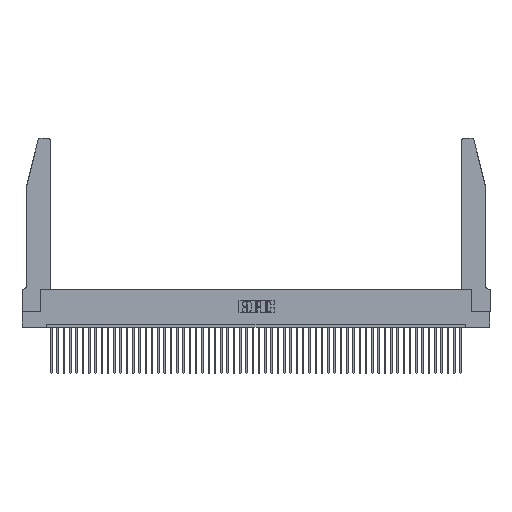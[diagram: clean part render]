
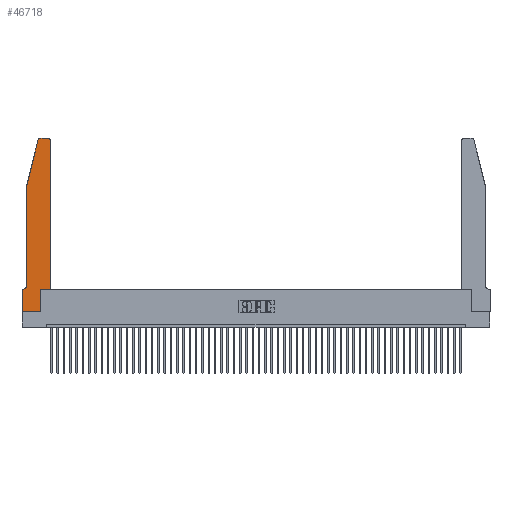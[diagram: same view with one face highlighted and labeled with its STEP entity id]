
A CAD part, top view. The second image highlights one B-rep face of the part: STEP entity #46718.
In plain terms, the highlighted planar face has unit normal (0, 0, 1).
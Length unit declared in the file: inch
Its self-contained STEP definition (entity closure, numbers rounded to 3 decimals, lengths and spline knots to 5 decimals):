
#19 = DIRECTION ( 'NONE',  ( 0., 0., 1. ) ) ;
#171 = EDGE_CURVE ( 'NONE', #25210, #6181, #39490, .T. ) ;
#871 = CARTESIAN_POINT ( 'NONE',  ( 0.2865, 0.35, 0.37 ) ) ;
#1043 = DIRECTION ( 'NONE',  ( 0., 1., 0. ) ) ;
#1110 = VERTEX_POINT ( 'NONE', #12302 ) ;
#1842 = ORIENTED_EDGE ( 'NONE', *, *, #15067, .T. ) ;
#2196 = CARTESIAN_POINT ( 'NONE',  ( 0., 0.35, 0.37 ) ) ;
#2297 = VECTOR ( 'NONE', #5967, 39.37008 ) ;
#3473 = LINE ( 'NONE', #14697, #22764 ) ;
#3910 = DIRECTION ( 'NONE',  ( 0., -1., 0. ) ) ;
#4078 = ORIENTED_EDGE ( 'NONE', *, *, #33581, .T. ) ;
#4260 = EDGE_CURVE ( 'NONE', #44697, #17746, #29826, .T. ) ;
#4726 = CARTESIAN_POINT ( 'NONE',  ( 0., 0., 0.37 ) ) ;
#5235 = VERTEX_POINT ( 'NONE', #29947 ) ;
#5526 = DIRECTION ( 'NONE',  ( 1., 0., 0. ) ) ;
#5967 = DIRECTION ( 'NONE',  ( -1., 0., 0. ) ) ;
#6181 = VERTEX_POINT ( 'NONE', #27707 ) ;
#7035 = ORIENTED_EDGE ( 'NONE', *, *, #21405, .T. ) ;
#7250 = EDGE_CURVE ( 'NONE', #1110, #44697, #3473, .T. ) ;
#7410 = VECTOR ( 'NONE', #10769, 39.37008 ) ;
#8171 = DIRECTION ( 'NONE',  ( 1., 0., 0. ) ) ;
#8192 = CARTESIAN_POINT ( 'NONE',  ( 0.4505, 0.35, 0.37 ) ) ;
#9369 = DIRECTION ( 'NONE',  ( 0., 1., 0. ) ) ;
#9827 = VECTOR ( 'NONE', #3910, 39.37008 ) ;
#10769 = DIRECTION ( 'NONE',  ( 1., 0., 0. ) ) ;
#12302 = CARTESIAN_POINT ( 'NONE',  ( 0.0055, 0.35, 0.37 ) ) ;
#13130 = CARTESIAN_POINT ( 'NONE',  ( 0.0055, 0.42, 0.37 ) ) ;
#13409 = CARTESIAN_POINT ( 'NONE',  ( 0.0755, 2., 0.37 ) ) ;
#13596 = CARTESIAN_POINT ( 'NONE',  ( 0., 0., 0.37 ) ) ;
#13872 = ORIENTED_EDGE ( 'NONE', *, *, #24236, .T. ) ;
#14280 = CARTESIAN_POINT ( 'NONE',  ( 0.2605, 2.75, 0.37 ) ) ;
#14697 = CARTESIAN_POINT ( 'NONE',  ( 0.0755, 0.35, 0.37 ) ) ;
#15067 = EDGE_CURVE ( 'NONE', #46160, #40145, #40225, .T. ) ;
#15393 = CIRCLE ( 'NONE', #32398, 0.07 ) ;
#15553 = VERTEX_POINT ( 'NONE', #37502 ) ;
#15912 = CARTESIAN_POINT ( 'NONE',  ( 0., 0.35, 0.37 ) ) ;
#16019 = EDGE_CURVE ( 'NONE', #15553, #5235, #30978, .T. ) ;
#16510 = LINE ( 'NONE', #41468, #25239 ) ;
#16711 = VERTEX_POINT ( 'NONE', #38688 ) ;
#17746 = VERTEX_POINT ( 'NONE', #13596 ) ;
#18865 = LINE ( 'NONE', #871, #36101 ) ;
#19249 = AXIS2_PLACEMENT_3D ( 'NONE', #21527, #39036, #47330 ) ;
#19499 = CARTESIAN_POINT ( 'NONE',  ( 0.25487, 2.72718, 0.37 ) ) ;
#20459 = ORIENTED_EDGE ( 'NONE', *, *, #16019, .T. ) ;
#20524 = EDGE_LOOP ( 'NONE', ( #37346, #1842, #40385, #47467, #13872, #21397, #48503, #25365, #7035, #20459, #44644, #4078 ) ) ;
#20761 = DIRECTION ( 'NONE',  ( 0., 0., -1. ) ) ;
#20930 = DIRECTION ( 'NONE',  ( -1., 0., 0. ) ) ;
#21397 = ORIENTED_EDGE ( 'NONE', *, *, #7250, .T. ) ;
#21405 = EDGE_CURVE ( 'NONE', #16711, #15553, #18865, .T. ) ;
#21527 = CARTESIAN_POINT ( 'NONE',  ( 0.4205, 2.72, 0.37 ) ) ;
#22764 = VECTOR ( 'NONE', #42815, 39.37008 ) ;
#23210 = AXIS2_PLACEMENT_3D ( 'NONE', #28275, #47425, #8171 ) ;
#24236 = EDGE_CURVE ( 'NONE', #6181, #1110, #15393, .T. ) ;
#25042 = DIRECTION ( 'NONE',  ( -0.239, -0.971, 0. ) ) ;
#25148 = CARTESIAN_POINT ( 'NONE',  ( 0.284, 2.75, 0.37 ) ) ;
#25210 = VERTEX_POINT ( 'NONE', #39870 ) ;
#25239 = VECTOR ( 'NONE', #5526, 39.37008 ) ;
#25365 = ORIENTED_EDGE ( 'NONE', *, *, #25664, .T. ) ;
#25664 = EDGE_CURVE ( 'NONE', #17746, #16711, #16510, .T. ) ;
#26647 = CARTESIAN_POINT ( 'NONE',  ( 0.4205, 2.75, 0.37 ) ) ;
#26898 = EDGE_CURVE ( 'NONE', #5235, #47014, #45210, .T. ) ;
#27395 = VERTEX_POINT ( 'NONE', #26647 ) ;
#27707 = CARTESIAN_POINT ( 'NONE',  ( 0.0755, 0.42, 0.37 ) ) ;
#27878 = PLANE ( 'NONE',  #34518 ) ;
#28043 = DIRECTION ( 'NONE',  ( 1., 0., 0. ) ) ;
#28275 = CARTESIAN_POINT ( 'NONE',  ( 0.284, 2.72, 0.37 ) ) ;
#28804 = FACE_OUTER_BOUND ( 'NONE', #20524, .T. ) ;
#29826 = LINE ( 'NONE', #4726, #40233 ) ;
#29947 = CARTESIAN_POINT ( 'NONE',  ( 0.4505, 0.35, 0.37 ) ) ;
#30978 = LINE ( 'NONE', #38572, #7410 ) ;
#32398 = AXIS2_PLACEMENT_3D ( 'NONE', #13130, #20761, #20930 ) ;
#33581 = EDGE_CURVE ( 'NONE', #47014, #27395, #39062, .T. ) ;
#34518 = AXIS2_PLACEMENT_3D ( 'NONE', #15912, #19, #28043 ) ;
#34811 = VECTOR ( 'NONE', #9369, 39.37008 ) ;
#36101 = VECTOR ( 'NONE', #1043, 39.37008 ) ;
#37346 = ORIENTED_EDGE ( 'NONE', *, *, #45717, .T. ) ;
#37467 = CARTESIAN_POINT ( 'NONE',  ( 0.4505, 2.72, 0.37 ) ) ;
#37502 = CARTESIAN_POINT ( 'NONE',  ( 0.2865, 0.35, 0.37 ) ) ;
#38572 = CARTESIAN_POINT ( 'NONE',  ( 0.4505, 0.35, 0.37 ) ) ;
#38688 = CARTESIAN_POINT ( 'NONE',  ( 0.2865, 0., 0.37 ) ) ;
#38995 = CARTESIAN_POINT ( 'NONE',  ( 0.0755, 2., 0.37 ) ) ;
#39036 = DIRECTION ( 'NONE',  ( 0., 0., 1. ) ) ;
#39062 = CIRCLE ( 'NONE', #19249, 0.03 ) ;
#39490 = LINE ( 'NONE', #38995, #9827 ) ;
#39870 = CARTESIAN_POINT ( 'NONE',  ( 0.0755, 2., 0.37 ) ) ;
#40145 = VERTEX_POINT ( 'NONE', #19499 ) ;
#40225 = CIRCLE ( 'NONE', #23210, 0.03 ) ;
#40233 = VECTOR ( 'NONE', #44454, 39.37008 ) ;
#40385 = ORIENTED_EDGE ( 'NONE', *, *, #47408, .T. ) ;
#41468 = CARTESIAN_POINT ( 'NONE',  ( 0., 0., 0.37 ) ) ;
#42815 = DIRECTION ( 'NONE',  ( -1., 0., 0. ) ) ;
#42864 = VECTOR ( 'NONE', #25042, 39.37008 ) ;
#44296 = LINE ( 'NONE', #14280, #2297 ) ;
#44454 = DIRECTION ( 'NONE',  ( 0., -1., 0. ) ) ;
#44644 = ORIENTED_EDGE ( 'NONE', *, *, #26898, .T. ) ;
#44697 = VERTEX_POINT ( 'NONE', #2196 ) ;
#45210 = LINE ( 'NONE', #8192, #34811 ) ;
#45717 = EDGE_CURVE ( 'NONE', #27395, #46160, #44296, .T. ) ;
#46160 = VERTEX_POINT ( 'NONE', #25148 ) ;
#46572 = LINE ( 'NONE', #13409, #42864 ) ;
#46718 = ADVANCED_FACE ( 'NONE', ( #28804 ), #27878, .T. ) ;
#47014 = VERTEX_POINT ( 'NONE', #37467 ) ;
#47330 = DIRECTION ( 'NONE',  ( 1., 0., 0. ) ) ;
#47408 = EDGE_CURVE ( 'NONE', #40145, #25210, #46572, .T. ) ;
#47425 = DIRECTION ( 'NONE',  ( 0., 0., 1. ) ) ;
#47467 = ORIENTED_EDGE ( 'NONE', *, *, #171, .T. ) ;
#48503 = ORIENTED_EDGE ( 'NONE', *, *, #4260, .T. ) ;
